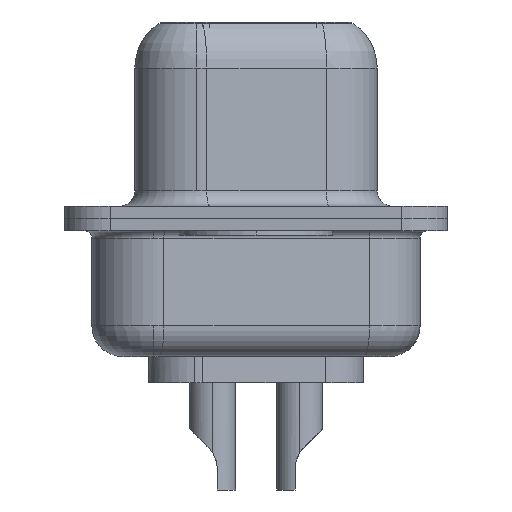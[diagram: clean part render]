
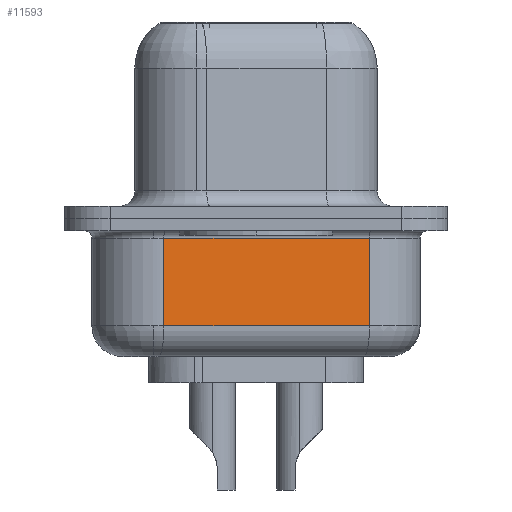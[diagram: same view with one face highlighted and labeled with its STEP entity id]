
A CAD part, left-side view. The second image highlights one B-rep face of the part: STEP entity #11593.
In plain terms, the highlighted planar face has unit normal (-0.985, -0.174, 0).
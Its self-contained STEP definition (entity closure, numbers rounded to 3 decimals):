
#280 = DIRECTION ( 'NONE',  ( 0., 0., 1. ) ) ;
#891 = VERTEX_POINT ( 'NONE', #6322 ) ;
#2231 = EDGE_CURVE ( 'NONE', #4139, #13975, #6195, .T. ) ;
#2280 = DIRECTION ( 'NONE',  ( -0.174, 0.985, 0. ) ) ;
#2927 = DIRECTION ( 'NONE',  ( 0., 0., 1. ) ) ;
#3630 = ORIENTED_EDGE ( 'NONE', *, *, #17670, .F. ) ;
#3793 = CARTESIAN_POINT ( 'NONE',  ( 2.855, 3.003, -0.65 ) ) ;
#3826 = LINE ( 'NONE', #13189, #4010 ) ;
#4010 = VECTOR ( 'NONE', #7101, 1000. ) ;
#4139 = VERTEX_POINT ( 'NONE', #16199 ) ;
#4462 = FACE_OUTER_BOUND ( 'NONE', #19944, .T. ) ;
#4675 = DIRECTION ( 'NONE',  ( -0.174, 0.985, 0. ) ) ;
#5221 = CARTESIAN_POINT ( 'NONE',  ( 4.037, -3.697, -0.65 ) ) ;
#6195 = LINE ( 'NONE', #7617, #16855 ) ;
#6254 = ORIENTED_EDGE ( 'NONE', *, *, #2231, .T. ) ;
#6322 = CARTESIAN_POINT ( 'NONE',  ( 2.855, 3.003, -3.5 ) ) ;
#7101 = DIRECTION ( 'NONE',  ( 0.174, -0.985, 0. ) ) ;
#7617 = CARTESIAN_POINT ( 'NONE',  ( 4.037, -3.697, -4.5 ) ) ;
#7733 = PLANE ( 'NONE',  #16072 ) ;
#9140 = EDGE_CURVE ( 'NONE', #891, #4139, #3826, .T. ) ;
#11593 = ADVANCED_FACE ( 'NONE', ( #4462 ), #7733, .F. ) ;
#11963 = VERTEX_POINT ( 'NONE', #15244 ) ;
#12109 = CARTESIAN_POINT ( 'NONE',  ( 2.855, 3.003, -4.5 ) ) ;
#12588 = CARTESIAN_POINT ( 'NONE',  ( 2.855, 3.003, -4.5 ) ) ;
#13189 = CARTESIAN_POINT ( 'NONE',  ( 2.855, 3.003, -3.5 ) ) ;
#13256 = ORIENTED_EDGE ( 'NONE', *, *, #9140, .T. ) ;
#13264 = LINE ( 'NONE', #3793, #15216 ) ;
#13975 = VERTEX_POINT ( 'NONE', #5221 ) ;
#14041 = EDGE_CURVE ( 'NONE', #13975, #11963, #13264, .T. ) ;
#15216 = VECTOR ( 'NONE', #2280, 1000. ) ;
#15244 = CARTESIAN_POINT ( 'NONE',  ( 2.855, 3.003, -0.65 ) ) ;
#15641 = LINE ( 'NONE', #12588, #18921 ) ;
#16072 = AXIS2_PLACEMENT_3D ( 'NONE', #12109, #18611, #4675 ) ;
#16199 = CARTESIAN_POINT ( 'NONE',  ( 4.037, -3.697, -3.5 ) ) ;
#16270 = ORIENTED_EDGE ( 'NONE', *, *, #14041, .T. ) ;
#16855 = VECTOR ( 'NONE', #2927, 1000. ) ;
#17670 = EDGE_CURVE ( 'NONE', #891, #11963, #15641, .T. ) ;
#18611 = DIRECTION ( 'NONE',  ( 0.985, 0.174, 0. ) ) ;
#18921 = VECTOR ( 'NONE', #280, 1000. ) ;
#19944 = EDGE_LOOP ( 'NONE', ( #3630, #13256, #6254, #16270 ) ) ;
